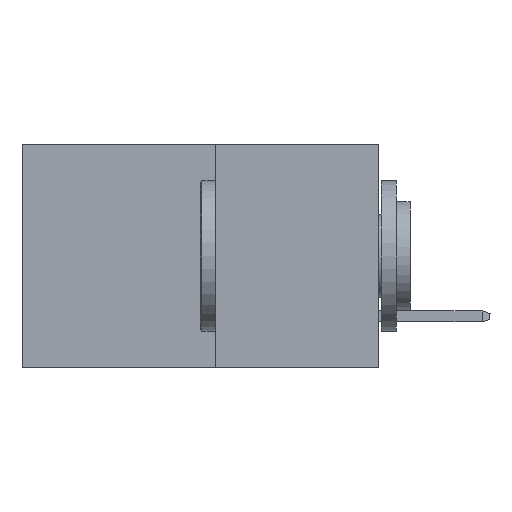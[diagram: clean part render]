
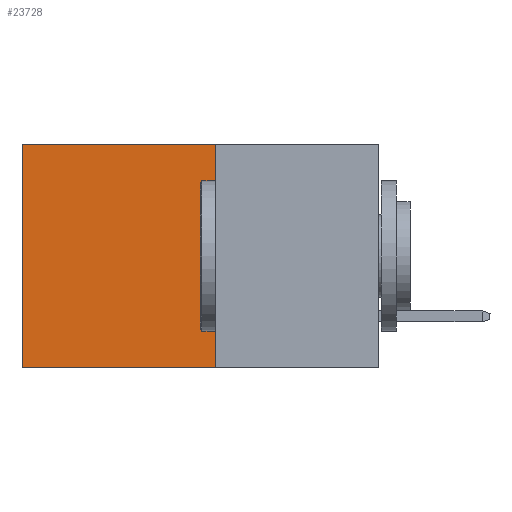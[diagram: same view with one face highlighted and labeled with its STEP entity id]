
A CAD part, left-side view. The second image highlights one B-rep face of the part: STEP entity #23728.
In plain terms, the highlighted planar face has unit normal (-1, 0, 0).
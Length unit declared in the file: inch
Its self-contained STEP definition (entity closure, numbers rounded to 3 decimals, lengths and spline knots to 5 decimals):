
#147 = AXIS2_PLACEMENT_3D ( 'NONE', #11708, #2308, #15528 ) ;
#1660 = CARTESIAN_POINT ( 'NONE',  ( 0.277, 0.59, -0.37 ) ) ;
#2308 = DIRECTION ( 'NONE',  ( 1., 0., 0. ) ) ;
#2389 = LINE ( 'NONE', #6908, #21848 ) ;
#2601 = VERTEX_POINT ( 'NONE', #17523 ) ;
#3171 = EDGE_CURVE ( 'NONE', #2601, #9200, #2389, .T. ) ;
#4908 = DIRECTION ( 'NONE',  ( 0., 0., -1. ) ) ;
#5998 = EDGE_CURVE ( 'NONE', #11755, #9509, #11805, .T. ) ;
#6777 = DIRECTION ( 'NONE',  ( 0., 1., 0. ) ) ;
#6833 = CARTESIAN_POINT ( 'NONE',  ( 0.277, 0.27, -0.37 ) ) ;
#6908 = CARTESIAN_POINT ( 'NONE',  ( 0.277, 0.27, -0.37 ) ) ;
#7580 = EDGE_CURVE ( 'NONE', #9509, #9200, #20008, .T. ) ;
#8107 = ORIENTED_EDGE ( 'NONE', *, *, #9031, .F. ) ;
#8270 = CARTESIAN_POINT ( 'NONE',  ( 0.277, 0.59, 0. ) ) ;
#9031 = EDGE_CURVE ( 'NONE', #11755, #2601, #23721, .T. ) ;
#9200 = VERTEX_POINT ( 'NONE', #1660 ) ;
#9509 = VERTEX_POINT ( 'NONE', #8270 ) ;
#11708 = CARTESIAN_POINT ( 'NONE',  ( 0.277, 0.27, -0.37 ) ) ;
#11755 = VERTEX_POINT ( 'NONE', #16220 ) ;
#11805 = LINE ( 'NONE', #22228, #17475 ) ;
#12427 = CARTESIAN_POINT ( 'NONE',  ( 0.277, 0.59, -0.37 ) ) ;
#12861 = ORIENTED_EDGE ( 'NONE', *, *, #7580, .T. ) ;
#13708 = VECTOR ( 'NONE', #23796, 39.37008 ) ;
#14986 = VECTOR ( 'NONE', #4908, 39.37008 ) ;
#15528 = DIRECTION ( 'NONE',  ( 0., 0., -1. ) ) ;
#16220 = CARTESIAN_POINT ( 'NONE',  ( 0.277, 0.27, 0. ) ) ;
#16738 = FACE_OUTER_BOUND ( 'NONE', #18222, .T. ) ;
#17475 = VECTOR ( 'NONE', #21994, 39.37008 ) ;
#17523 = CARTESIAN_POINT ( 'NONE',  ( 0.277, 0.27, -0.37 ) ) ;
#17666 = ORIENTED_EDGE ( 'NONE', *, *, #3171, .F. ) ;
#18222 = EDGE_LOOP ( 'NONE', ( #12861, #17666, #8107, #18255 ) ) ;
#18255 = ORIENTED_EDGE ( 'NONE', *, *, #5998, .T. ) ;
#20008 = LINE ( 'NONE', #12427, #14986 ) ;
#21848 = VECTOR ( 'NONE', #6777, 39.37008 ) ;
#21994 = DIRECTION ( 'NONE',  ( 0., 1., 0. ) ) ;
#22228 = CARTESIAN_POINT ( 'NONE',  ( 0.277, 0.27, 0. ) ) ;
#22987 = PLANE ( 'NONE',  #147 ) ;
#23721 = LINE ( 'NONE', #6833, #13708 ) ;
#23728 = ADVANCED_FACE ( 'NONE', ( #16738 ), #22987, .F. ) ;
#23796 = DIRECTION ( 'NONE',  ( 0., 0., -1. ) ) ;
